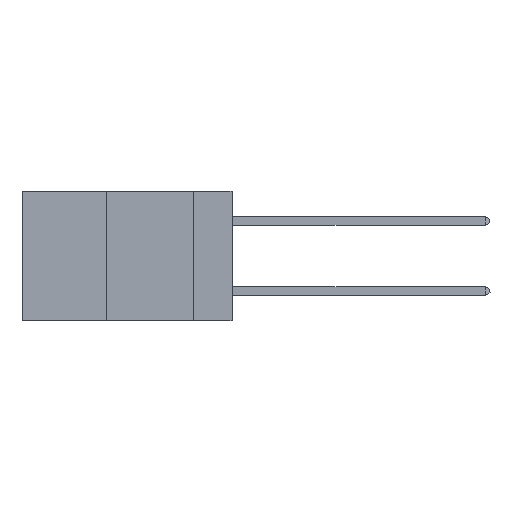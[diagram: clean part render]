
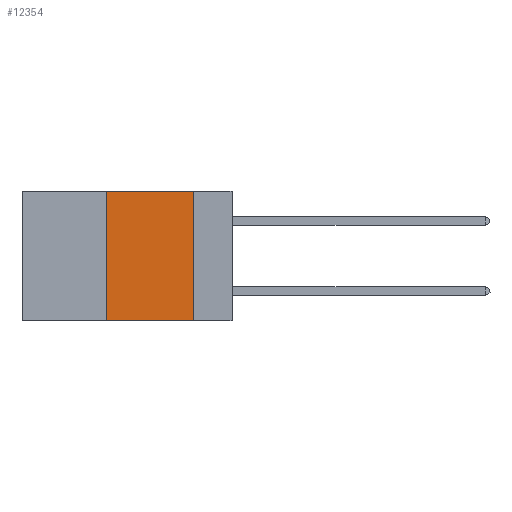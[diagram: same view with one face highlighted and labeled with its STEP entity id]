
A CAD part, left-side view. The second image highlights one B-rep face of the part: STEP entity #12354.
In plain terms, the highlighted planar face has unit normal (-1, 0, 0).
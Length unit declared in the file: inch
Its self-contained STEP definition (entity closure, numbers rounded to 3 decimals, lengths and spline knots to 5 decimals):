
#30 = DIRECTION ( 'NONE',  ( 1., 0., 0. ) ) ;
#151 = DIRECTION ( 'NONE',  ( 0., 0., 1. ) ) ;
#826 = CARTESIAN_POINT ( 'NONE',  ( 0., 0.6, 0. ) ) ;
#1198 = VERTEX_POINT ( 'NONE', #2620 ) ;
#1643 = VERTEX_POINT ( 'NONE', #7400 ) ;
#2262 = FACE_OUTER_BOUND ( 'NONE', #5940, .T. ) ;
#2620 = CARTESIAN_POINT ( 'NONE',  ( 0., 0.36, -0.37 ) ) ;
#3037 = EDGE_CURVE ( 'NONE', #1643, #3814, #10775, .T. ) ;
#3471 = DIRECTION ( 'NONE',  ( 0., 0., -1. ) ) ;
#3564 = VECTOR ( 'NONE', #6388, 39.37008 ) ;
#3565 = PLANE ( 'NONE',  #11039 ) ;
#3613 = CARTESIAN_POINT ( 'NONE',  ( 0., 0.6, -0.37 ) ) ;
#3814 = VERTEX_POINT ( 'NONE', #8335 ) ;
#4665 = VERTEX_POINT ( 'NONE', #11725 ) ;
#5656 = LINE ( 'NONE', #6904, #6884 ) ;
#5920 = ORIENTED_EDGE ( 'NONE', *, *, #3037, .F. ) ;
#5940 = EDGE_LOOP ( 'NONE', ( #6712, #5920, #10152, #10348 ) ) ;
#6388 = DIRECTION ( 'NONE',  ( 0., -1., 0. ) ) ;
#6712 = ORIENTED_EDGE ( 'NONE', *, *, #14487, .F. ) ;
#6884 = VECTOR ( 'NONE', #3471, 39.37008 ) ;
#6904 = CARTESIAN_POINT ( 'NONE',  ( 0., 0.11, 0. ) ) ;
#7299 = VECTOR ( 'NONE', #13851, 39.37008 ) ;
#7400 = CARTESIAN_POINT ( 'NONE',  ( 0., 0.36, 0. ) ) ;
#7510 = EDGE_CURVE ( 'NONE', #1198, #4665, #13703, .T. ) ;
#7857 = LINE ( 'NONE', #10194, #10642 ) ;
#8335 = CARTESIAN_POINT ( 'NONE',  ( 0., 0.11, 0. ) ) ;
#10152 = ORIENTED_EDGE ( 'NONE', *, *, #14460, .F. ) ;
#10194 = CARTESIAN_POINT ( 'NONE',  ( 0., 0.36, 0. ) ) ;
#10348 = ORIENTED_EDGE ( 'NONE', *, *, #7510, .T. ) ;
#10642 = VECTOR ( 'NONE', #151, 39.37008 ) ;
#10775 = LINE ( 'NONE', #826, #3564 ) ;
#11039 = AXIS2_PLACEMENT_3D ( 'NONE', #12198, #30, #13444 ) ;
#11725 = CARTESIAN_POINT ( 'NONE',  ( 0., 0.11, -0.37 ) ) ;
#12198 = CARTESIAN_POINT ( 'NONE',  ( 0., 0.6, 0. ) ) ;
#12354 = ADVANCED_FACE ( 'NONE', ( #2262 ), #3565, .F. ) ;
#13444 = DIRECTION ( 'NONE',  ( 0., 0., -1. ) ) ;
#13703 = LINE ( 'NONE', #3613, #7299 ) ;
#13851 = DIRECTION ( 'NONE',  ( 0., -1., 0. ) ) ;
#14460 = EDGE_CURVE ( 'NONE', #1198, #1643, #7857, .T. ) ;
#14487 = EDGE_CURVE ( 'NONE', #3814, #4665, #5656, .T. ) ;
